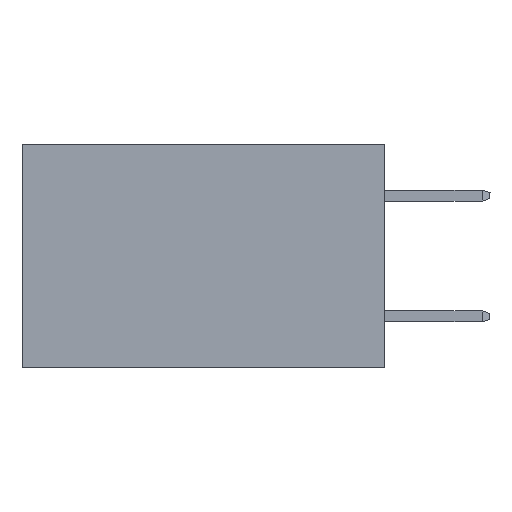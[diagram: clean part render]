
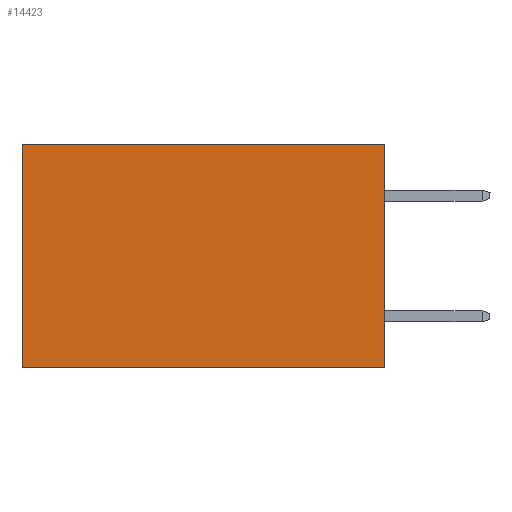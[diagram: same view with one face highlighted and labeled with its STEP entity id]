
A CAD part, left-side view. The second image highlights one B-rep face of the part: STEP entity #14423.
In plain terms, the highlighted planar face has unit normal (-1, 0, 0).
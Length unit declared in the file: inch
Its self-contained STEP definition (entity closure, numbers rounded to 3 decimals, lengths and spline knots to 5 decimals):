
#759 = CARTESIAN_POINT ( 'NONE',  ( 0.298, 0., 0. ) ) ;
#1231 = DIRECTION ( 'NONE',  ( 0., 1., 0. ) ) ;
#3064 = DIRECTION ( 'NONE',  ( 0., 0., -1. ) ) ;
#4099 = LINE ( 'NONE', #759, #29467 ) ;
#4789 = EDGE_CURVE ( 'NONE', #23034, #28170, #8128, .T. ) ;
#5454 = LINE ( 'NONE', #18145, #14741 ) ;
#6795 = ORIENTED_EDGE ( 'NONE', *, *, #13184, .F. ) ;
#8128 = LINE ( 'NONE', #14576, #27315 ) ;
#8405 = CARTESIAN_POINT ( 'NONE',  ( 0.298, 0.6, 0. ) ) ;
#9274 = DIRECTION ( 'NONE',  ( 1., 0., 0. ) ) ;
#9380 = DIRECTION ( 'NONE',  ( 0., 0., -1. ) ) ;
#9585 = CARTESIAN_POINT ( 'NONE',  ( 0.298, 0., -0.37 ) ) ;
#9943 = VECTOR ( 'NONE', #9380, 39.37008 ) ;
#11440 = PLANE ( 'NONE',  #17319 ) ;
#13184 = EDGE_CURVE ( 'NONE', #13438, #23034, #4099, .T. ) ;
#13438 = VERTEX_POINT ( 'NONE', #26246 ) ;
#14423 = ADVANCED_FACE ( 'NONE', ( #31270 ), #11440, .F. ) ;
#14576 = CARTESIAN_POINT ( 'NONE',  ( 0.298, 0., -0.37 ) ) ;
#14741 = VECTOR ( 'NONE', #1231, 39.37008 ) ;
#14953 = LINE ( 'NONE', #31637, #9943 ) ;
#15817 = CARTESIAN_POINT ( 'NONE',  ( 0.298, 0.6, -0.37 ) ) ;
#16577 = DIRECTION ( 'NONE',  ( 0., 0., -1. ) ) ;
#17319 = AXIS2_PLACEMENT_3D ( 'NONE', #28547, #9274, #16577 ) ;
#18145 = CARTESIAN_POINT ( 'NONE',  ( 0.298, 0., 0. ) ) ;
#20222 = EDGE_CURVE ( 'NONE', #27575, #28170, #14953, .T. ) ;
#21676 = EDGE_LOOP ( 'NONE', ( #31063, #28145, #6795, #23257 ) ) ;
#22077 = DIRECTION ( 'NONE',  ( 0., 1., 0. ) ) ;
#23034 = VERTEX_POINT ( 'NONE', #9585 ) ;
#23257 = ORIENTED_EDGE ( 'NONE', *, *, #23658, .T. ) ;
#23658 = EDGE_CURVE ( 'NONE', #13438, #27575, #5454, .T. ) ;
#26246 = CARTESIAN_POINT ( 'NONE',  ( 0.298, 0., 0. ) ) ;
#27315 = VECTOR ( 'NONE', #22077, 39.37008 ) ;
#27575 = VERTEX_POINT ( 'NONE', #8405 ) ;
#28145 = ORIENTED_EDGE ( 'NONE', *, *, #4789, .F. ) ;
#28170 = VERTEX_POINT ( 'NONE', #15817 ) ;
#28547 = CARTESIAN_POINT ( 'NONE',  ( 0.298, 0., 0. ) ) ;
#29467 = VECTOR ( 'NONE', #3064, 39.37008 ) ;
#31063 = ORIENTED_EDGE ( 'NONE', *, *, #20222, .T. ) ;
#31270 = FACE_OUTER_BOUND ( 'NONE', #21676, .T. ) ;
#31637 = CARTESIAN_POINT ( 'NONE',  ( 0.298, 0.6, 0. ) ) ;
